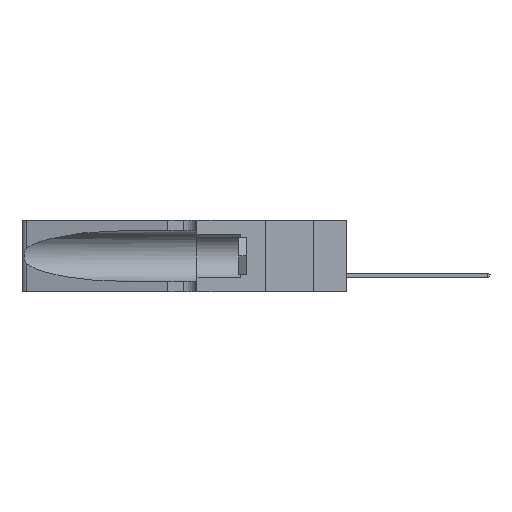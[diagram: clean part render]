
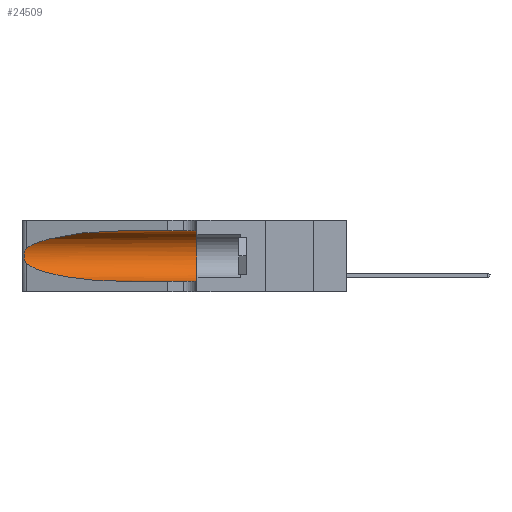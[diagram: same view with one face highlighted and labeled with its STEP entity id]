
A CAD part, left-side view. The second image highlights one B-rep face of the part: STEP entity #24509.
In plain terms, the highlighted cylindrical face has radius 3.308 mm (diameter 6.617 mm), a partial arc.
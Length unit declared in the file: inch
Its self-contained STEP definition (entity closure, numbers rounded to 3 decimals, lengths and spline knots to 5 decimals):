
#241 = CARTESIAN_POINT ( 'NONE',  ( 0.25639, 1.23186, 0.15144 ) ) ;
#564 = EDGE_CURVE ( 'NONE', #29185, #31399, #23378, .T. ) ;
#581 = VERTEX_POINT ( 'NONE', #23785 ) ;
#626 = CARTESIAN_POINT ( 'NONE',  ( 0.25555, 1.22994, 0.2215 ) ) ;
#2407 = ORIENTED_EDGE ( 'NONE', *, *, #4431, .T. ) ;
#2411 = CARTESIAN_POINT ( 'NONE',  ( 0.1305, 0.72297, 0.05475 ) ) ;
#2810 = DIRECTION ( 'NONE',  ( 0., 0., 1. ) ) ;
#3240 = ORIENTED_EDGE ( 'NONE', *, *, #10219, .T. ) ;
#3270 = CARTESIAN_POINT ( 'NONE',  ( 0.25555, 1.22993, 0.14849 ) ) ;
#3401 = CARTESIAN_POINT ( 'NONE',  ( 0.26075, 1.23896, 0.19203 ) ) ;
#3517 = CARTESIAN_POINT ( 'NONE',  ( 0.25639, 1.23184, 0.21858 ) ) ;
#3672 = LINE ( 'NONE', #35417, #31827 ) ;
#4431 = EDGE_CURVE ( 'NONE', #581, #31298, #29725, .T. ) ;
#4831 = CARTESIAN_POINT ( 'NONE',  ( 0.2373, 1.15595, 0.28018 ) ) ;
#5403 = CARTESIAN_POINT ( 'NONE',  ( 0.18966, 0.96281, 0.05475 ) ) ;
#5497 = CARTESIAN_POINT ( 'NONE',  ( 0.1305, 0.72297, 0.31525 ) ) ;
#5969 = AXIS2_PLACEMENT_3D ( 'NONE', #12828, #10061, #22289 ) ;
#6311 = VERTEX_POINT ( 'NONE', #38028 ) ;
#6403 = VECTOR ( 'NONE', #11315, 39.37008 ) ;
#7127 = CARTESIAN_POINT ( 'NONE',  ( 0.1305, 0.35, 0.05475 ) ) ;
#7300 = ORIENTED_EDGE ( 'NONE', *, *, #564, .T. ) ;
#8811 = CARTESIAN_POINT ( 'NONE',  ( 0.25487, 1.22718, 0.22369 ) ) ;
#9158 = CARTESIAN_POINT ( 'NONE',  ( 0.25789, 1.23486, 0.15765 ) ) ;
#9392 = CARTESIAN_POINT ( 'NONE',  ( 0.26018, 1.23835, 0.19895 ) ) ;
#10061 = DIRECTION ( 'NONE',  ( 0., -1., 0. ) ) ;
#10219 = EDGE_CURVE ( 'NONE', #31298, #29185, #26838, .T. ) ;
#11138 = EDGE_CURVE ( 'NONE', #26678, #6311, #3672, .T. ) ;
#11315 = DIRECTION ( 'NONE',  ( 0., -1., 0. ) ) ;
#12828 = CARTESIAN_POINT ( 'NONE',  ( 0.1305, 1.61858, 0.185 ) ) ;
#14371 = DIRECTION ( 'NONE',  ( 0., 1., 0. ) ) ;
#14608 = CYLINDRICAL_SURFACE ( 'NONE', #5969, 0.13025 ) ;
#15316 = CARTESIAN_POINT ( 'NONE',  ( 0.25487, 1.22718, 0.14631 ) ) ;
#15383 = CARTESIAN_POINT ( 'NONE',  ( 0.25487, 1.22718, 0.14631 ) ) ;
#16337 = ORIENTED_EDGE ( 'NONE', *, *, #30550, .T. ) ;
#17243 = CARTESIAN_POINT ( 'NONE',  ( 0.1305, 1.61858, 0.05475 ) ) ;
#17417 = DIRECTION ( 'NONE',  ( 0., -1., 0. ) ) ;
#17627 = CARTESIAN_POINT ( 'NONE',  ( 0.1305, 0.35, 0.185 ) ) ;
#18218 = CARTESIAN_POINT ( 'NONE',  ( 0.26075, 1.23896, 0.178 ) ) ;
#19798 = CARTESIAN_POINT ( 'NONE',  ( 0.18966, 0.96281, 0.31525 ) ) ;
#21736 = CARTESIAN_POINT ( 'NONE',  ( 0.25787, 1.23484, 0.2124 ) ) ;
#22289 = DIRECTION ( 'NONE',  ( 0., 0., -1. ) ) ;
#22810 = CARTESIAN_POINT ( 'NONE',  ( 0.25487, 1.22718, 0.22369 ) ) ;
#22971 = CARTESIAN_POINT ( 'NONE',  ( 0.25487, 1.22718, 0.14631 ) ) ;
#23378 = LINE ( 'NONE', #17243, #6403 ) ;
#23785 = CARTESIAN_POINT ( 'NONE',  ( 0.25487, 1.22718, 0.22369 ) ) ;
#24435 = FACE_OUTER_BOUND ( 'NONE', #33608, .T. ) ;
#24509 = ADVANCED_FACE ( 'NONE', ( #24435 ), #14608, .F. ) ;
#24779 = CARTESIAN_POINT ( 'NONE',  ( 0.26017, 1.23833, 0.17102 ) ) ;
#26678 = VERTEX_POINT ( 'NONE', #5497 ) ;
#26838 =( BOUNDED_CURVE ( )  B_SPLINE_CURVE ( 3, ( #22971, #32014, #5403, #2411 ),
 .UNSPECIFIED., .F., .T. ) 
 B_SPLINE_CURVE_WITH_KNOTS ( ( 4, 4 ),
 ( 3.44316, 4.71239 ),
 .UNSPECIFIED. ) 
 CURVE ( )  GEOMETRIC_REPRESENTATION_ITEM ( )  RATIONAL_B_SPLINE_CURVE ( ( 1., 0.87, 0.87, 1. ) ) 
 REPRESENTATION_ITEM ( '' )  );
#29185 = VERTEX_POINT ( 'NONE', #31028 ) ;
#29725 = B_SPLINE_CURVE_WITH_KNOTS ( 'NONE', 3,
 ( #8811, #626, #3517, #21736, #33268, #9392, #3401, #18218, #24779, #30395, #9158, #241, #3270, #15316 ),
 .UNSPECIFIED., .F., .F.,
 ( 4, 2, 2, 2, 2, 2, 4 ),
 ( 0., 0.00027, 0.00053, 0.00107, 0.0016, 0.00187, 0.00214 ),
 .UNSPECIFIED. ) ;
#30079 = ORIENTED_EDGE ( 'NONE', *, *, #11138, .F. ) ;
#30395 = CARTESIAN_POINT ( 'NONE',  ( 0.25856, 1.23593, 0.16098 ) ) ;
#30550 = EDGE_CURVE ( 'NONE', #26678, #581, #38383, .T. ) ;
#31028 = CARTESIAN_POINT ( 'NONE',  ( 0.1305, 0.72297, 0.05475 ) ) ;
#31298 = VERTEX_POINT ( 'NONE', #15383 ) ;
#31399 = VERTEX_POINT ( 'NONE', #7127 ) ;
#31827 = VECTOR ( 'NONE', #17417, 39.37008 ) ;
#32014 = CARTESIAN_POINT ( 'NONE',  ( 0.2373, 1.15595, 0.08982 ) ) ;
#32800 = CIRCLE ( 'NONE', #37027, 0.13025 ) ;
#33268 = CARTESIAN_POINT ( 'NONE',  ( 0.25854, 1.2359, 0.20912 ) ) ;
#33608 = EDGE_LOOP ( 'NONE', ( #16337, #2407, #3240, #7300, #38752, #30079 ) ) ;
#35417 = CARTESIAN_POINT ( 'NONE',  ( 0.1305, 1.61858, 0.31525 ) ) ;
#37027 = AXIS2_PLACEMENT_3D ( 'NONE', #17627, #14371, #2810 ) ;
#37779 = CARTESIAN_POINT ( 'NONE',  ( 0.1305, 0.72297, 0.31525 ) ) ;
#37878 = EDGE_CURVE ( 'NONE', #6311, #31399, #32800, .T. ) ;
#38028 = CARTESIAN_POINT ( 'NONE',  ( 0.1305, 0.35, 0.31525 ) ) ;
#38383 =( BOUNDED_CURVE ( )  B_SPLINE_CURVE ( 3, ( #37779, #19798, #4831, #22810 ),
 .UNSPECIFIED., .F., .T. ) 
 B_SPLINE_CURVE_WITH_KNOTS ( ( 4, 4 ),
 ( 1.5708, 2.84003 ),
 .UNSPECIFIED. ) 
 CURVE ( )  GEOMETRIC_REPRESENTATION_ITEM ( )  RATIONAL_B_SPLINE_CURVE ( ( 1., 0.87, 0.87, 1. ) ) 
 REPRESENTATION_ITEM ( '' )  );
#38752 = ORIENTED_EDGE ( 'NONE', *, *, #37878, .F. ) ;
